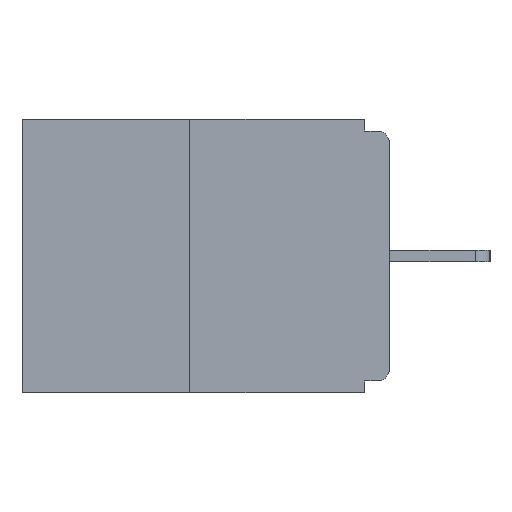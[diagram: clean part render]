
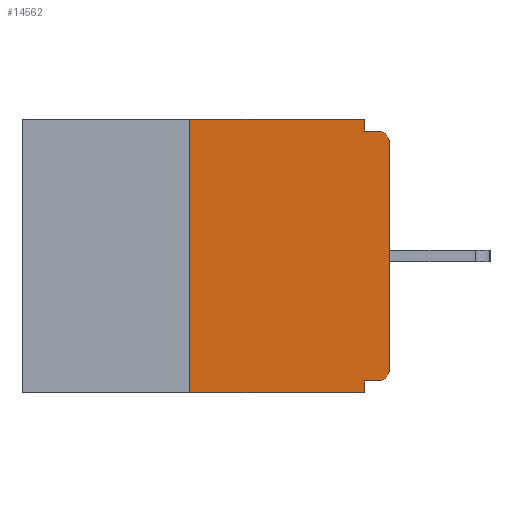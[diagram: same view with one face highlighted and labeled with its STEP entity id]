
A CAD part, left-side view. The second image highlights one B-rep face of the part: STEP entity #14562.
In plain terms, the highlighted planar face has unit normal (-1, 0, 0).
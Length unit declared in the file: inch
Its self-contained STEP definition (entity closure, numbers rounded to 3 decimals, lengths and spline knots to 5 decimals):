
#655 = ORIENTED_EDGE ( 'NONE', *, *, #14494, .F. ) ;
#729 = CIRCLE ( 'NONE', #11637, 0.015 ) ;
#761 = EDGE_CURVE ( 'NONE', #14356, #6094, #6181, .T. ) ;
#1112 = CARTESIAN_POINT ( 'NONE',  ( 0., 0.031, -0.328 ) ) ;
#2291 = EDGE_CURVE ( 'NONE', #17165, #14356, #4339, .T. ) ;
#2802 = VERTEX_POINT ( 'NONE', #16503 ) ;
#2980 = EDGE_CURVE ( 'NONE', #2802, #17165, #729, .T. ) ;
#3861 = EDGE_CURVE ( 'NONE', #8262, #21424, #11315, .T. ) ;
#4210 = DIRECTION ( 'NONE',  ( 0., 0., 1. ) ) ;
#4265 = VECTOR ( 'NONE', #8432, 39.37008 ) ;
#4339 = LINE ( 'NONE', #6182, #23197 ) ;
#4714 = ORIENTED_EDGE ( 'NONE', *, *, #2291, .T. ) ;
#4874 = EDGE_CURVE ( 'NONE', #16691, #21424, #16829, .T. ) ;
#5218 = CARTESIAN_POINT ( 'NONE',  ( 0., 0.015, -0.313 ) ) ;
#5282 = DIRECTION ( 'NONE',  ( 0., 0., -1. ) ) ;
#5424 = CARTESIAN_POINT ( 'NONE',  ( 0., 0.031, 0. ) ) ;
#5607 = DIRECTION ( 'NONE',  ( 0., 0., -1. ) ) ;
#5609 = CARTESIAN_POINT ( 'NONE',  ( 0., 0.25, 0. ) ) ;
#5616 = VECTOR ( 'NONE', #22391, 39.37008 ) ;
#5991 = FACE_OUTER_BOUND ( 'NONE', #18173, .T. ) ;
#6094 = VERTEX_POINT ( 'NONE', #7175 ) ;
#6181 = CIRCLE ( 'NONE', #17052, 0.015 ) ;
#6182 = CARTESIAN_POINT ( 'NONE',  ( 0., 0., 0. ) ) ;
#6549 = VERTEX_POINT ( 'NONE', #17380 ) ;
#7175 = CARTESIAN_POINT ( 'NONE',  ( 0., 0.015, -0.015 ) ) ;
#7966 = CARTESIAN_POINT ( 'NONE',  ( 0., 0.46, 0. ) ) ;
#8202 = CARTESIAN_POINT ( 'NONE',  ( 0., 0., -0.328 ) ) ;
#8262 = VERTEX_POINT ( 'NONE', #1112 ) ;
#8432 = DIRECTION ( 'NONE',  ( 0., -1., 0. ) ) ;
#8439 = CARTESIAN_POINT ( 'NONE',  ( 0., 0.031, -0.015 ) ) ;
#8693 = VECTOR ( 'NONE', #23439, 39.37008 ) ;
#8756 = CARTESIAN_POINT ( 'NONE',  ( 0., 0., -0.03 ) ) ;
#9827 = DIRECTION ( 'NONE',  ( 0., 0., -1. ) ) ;
#10396 = CARTESIAN_POINT ( 'NONE',  ( 0., 0.46, -0.343 ) ) ;
#10602 = EDGE_CURVE ( 'NONE', #6549, #17825, #25463, .T. ) ;
#11315 = LINE ( 'NONE', #23232, #22500 ) ;
#11607 = ORIENTED_EDGE ( 'NONE', *, *, #2980, .T. ) ;
#11637 = AXIS2_PLACEMENT_3D ( 'NONE', #5218, #13229, #5607 ) ;
#12457 = LINE ( 'NONE', #16641, #21267 ) ;
#12496 = ORIENTED_EDGE ( 'NONE', *, *, #761, .T. ) ;
#12580 = CARTESIAN_POINT ( 'NONE',  ( 0., 0., -0.313 ) ) ;
#12767 = EDGE_CURVE ( 'NONE', #2802, #8262, #20116, .T. ) ;
#13229 = DIRECTION ( 'NONE',  ( -1., 0., 0. ) ) ;
#14151 = PLANE ( 'NONE',  #25453 ) ;
#14304 = EDGE_CURVE ( 'NONE', #17825, #6094, #12457, .T. ) ;
#14356 = VERTEX_POINT ( 'NONE', #8756 ) ;
#14421 = VERTEX_POINT ( 'NONE', #5609 ) ;
#14494 = EDGE_CURVE ( 'NONE', #14421, #6549, #24997, .T. ) ;
#14514 = ORIENTED_EDGE ( 'NONE', *, *, #12767, .F. ) ;
#14562 = ADVANCED_FACE ( 'NONE', ( #5991 ), #14151, .F. ) ;
#14680 = DIRECTION ( 'NONE',  ( 0., -1., 0. ) ) ;
#14955 = LINE ( 'NONE', #24745, #5616 ) ;
#16210 = DIRECTION ( 'NONE',  ( 0., 1., 0. ) ) ;
#16231 = DIRECTION ( 'NONE',  ( 1., 0., 0. ) ) ;
#16503 = CARTESIAN_POINT ( 'NONE',  ( 0., 0.015, -0.328 ) ) ;
#16641 = CARTESIAN_POINT ( 'NONE',  ( 0., 0., -0.015 ) ) ;
#16691 = VERTEX_POINT ( 'NONE', #22548 ) ;
#16829 = LINE ( 'NONE', #10396, #4265 ) ;
#17052 = AXIS2_PLACEMENT_3D ( 'NONE', #19780, #24101, #9827 ) ;
#17165 = VERTEX_POINT ( 'NONE', #12580 ) ;
#17380 = CARTESIAN_POINT ( 'NONE',  ( 0., 0.031, 0. ) ) ;
#17825 = VERTEX_POINT ( 'NONE', #8439 ) ;
#17912 = DIRECTION ( 'NONE',  ( 0., 0., -1. ) ) ;
#18173 = EDGE_LOOP ( 'NONE', ( #655, #21045, #22559, #24749, #14514, #11607, #4714, #12496, #25670, #25089 ) ) ;
#18273 = VECTOR ( 'NONE', #16210, 39.37008 ) ;
#19780 = CARTESIAN_POINT ( 'NONE',  ( 0., 0.015, -0.03 ) ) ;
#20116 = LINE ( 'NONE', #8202, #18273 ) ;
#21045 = ORIENTED_EDGE ( 'NONE', *, *, #22087, .F. ) ;
#21267 = VECTOR ( 'NONE', #14680, 39.37008 ) ;
#21334 = CARTESIAN_POINT ( 'NONE',  ( 0., 0.46, 0. ) ) ;
#21424 = VERTEX_POINT ( 'NONE', #24841 ) ;
#22087 = EDGE_CURVE ( 'NONE', #16691, #14421, #14955, .T. ) ;
#22391 = DIRECTION ( 'NONE',  ( 0., 0., 1. ) ) ;
#22500 = VECTOR ( 'NONE', #5282, 39.37008 ) ;
#22548 = CARTESIAN_POINT ( 'NONE',  ( 0., 0.25, -0.343 ) ) ;
#22559 = ORIENTED_EDGE ( 'NONE', *, *, #4874, .T. ) ;
#22849 = VECTOR ( 'NONE', #25719, 39.37008 ) ;
#23197 = VECTOR ( 'NONE', #4210, 39.37008 ) ;
#23232 = CARTESIAN_POINT ( 'NONE',  ( 0., 0.031, -0.343 ) ) ;
#23439 = DIRECTION ( 'NONE',  ( 0., -1., 0. ) ) ;
#24101 = DIRECTION ( 'NONE',  ( -1., 0., 0. ) ) ;
#24745 = CARTESIAN_POINT ( 'NONE',  ( 0., 0.25, 0. ) ) ;
#24749 = ORIENTED_EDGE ( 'NONE', *, *, #3861, .F. ) ;
#24841 = CARTESIAN_POINT ( 'NONE',  ( 0., 0.031, -0.343 ) ) ;
#24997 = LINE ( 'NONE', #21334, #8693 ) ;
#25089 = ORIENTED_EDGE ( 'NONE', *, *, #10602, .F. ) ;
#25453 = AXIS2_PLACEMENT_3D ( 'NONE', #7966, #16231, #17912 ) ;
#25463 = LINE ( 'NONE', #5424, #22849 ) ;
#25670 = ORIENTED_EDGE ( 'NONE', *, *, #14304, .F. ) ;
#25719 = DIRECTION ( 'NONE',  ( 0., 0., -1. ) ) ;
